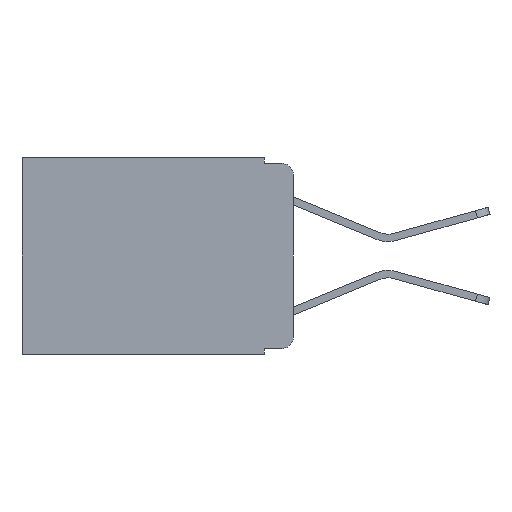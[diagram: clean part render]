
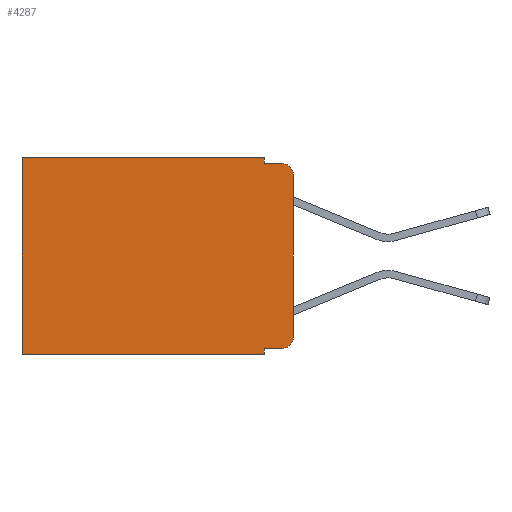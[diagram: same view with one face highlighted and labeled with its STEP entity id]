
A CAD part, left-side view. The second image highlights one B-rep face of the part: STEP entity #4287.
In plain terms, the highlighted planar face has unit normal (-1, 0, 0).
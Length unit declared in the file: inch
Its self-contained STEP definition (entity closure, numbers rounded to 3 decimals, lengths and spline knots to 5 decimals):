
#206 = CARTESIAN_POINT ( 'NONE',  ( 0.298, 0., -0.03 ) ) ;
#440 = CARTESIAN_POINT ( 'NONE',  ( 0.298, 0.051, 0. ) ) ;
#493 = VERTEX_POINT ( 'NONE', #10016 ) ;
#534 = AXIS2_PLACEMENT_3D ( 'NONE', #2322, #9544, #9946 ) ;
#638 = VECTOR ( 'NONE', #1713, 39.37008 ) ;
#674 = VECTOR ( 'NONE', #9344, 39.37008 ) ;
#797 = DIRECTION ( 'NONE',  ( 0., -1., 0. ) ) ;
#941 = DIRECTION ( 'NONE',  ( 0., 0., -1. ) ) ;
#974 = CARTESIAN_POINT ( 'NONE',  ( 0.298, 0.473, 0. ) ) ;
#1271 = EDGE_CURVE ( 'NONE', #8972, #6595, #2256, .T. ) ;
#1276 = VERTEX_POINT ( 'NONE', #10665 ) ;
#1374 = ORIENTED_EDGE ( 'NONE', *, *, #2510, .T. ) ;
#1549 = VECTOR ( 'NONE', #8406, 39.37008 ) ;
#1636 = ORIENTED_EDGE ( 'NONE', *, *, #2588, .F. ) ;
#1713 = DIRECTION ( 'NONE',  ( 0., 0., -1. ) ) ;
#1719 = VERTEX_POINT ( 'NONE', #5149 ) ;
#1764 = ORIENTED_EDGE ( 'NONE', *, *, #2994, .T. ) ;
#1784 = VERTEX_POINT ( 'NONE', #2625 ) ;
#1944 = EDGE_CURVE ( 'NONE', #493, #8972, #6693, .T. ) ;
#1969 = VECTOR ( 'NONE', #797, 39.37008 ) ;
#2031 = DIRECTION ( 'NONE',  ( 0., 0., -1. ) ) ;
#2215 = CARTESIAN_POINT ( 'NONE',  ( 0.298, 0.051, -0.01 ) ) ;
#2256 = CIRCLE ( 'NONE', #5093, 0.02 ) ;
#2265 = VERTEX_POINT ( 'NONE', #2926 ) ;
#2322 = CARTESIAN_POINT ( 'NONE',  ( 0.298, 0.02, -0.03 ) ) ;
#2338 = EDGE_CURVE ( 'NONE', #11211, #6595, #11148, .T. ) ;
#2438 = ORIENTED_EDGE ( 'NONE', *, *, #10673, .F. ) ;
#2510 = EDGE_CURVE ( 'NONE', #1276, #2265, #7933, .T. ) ;
#2533 = LINE ( 'NONE', #974, #4648 ) ;
#2588 = EDGE_CURVE ( 'NONE', #493, #5760, #6537, .T. ) ;
#2625 = CARTESIAN_POINT ( 'NONE',  ( 0.298, 0.051, -0.01 ) ) ;
#2793 = CARTESIAN_POINT ( 'NONE',  ( 0.298, 0.02, -0.333 ) ) ;
#2926 = CARTESIAN_POINT ( 'NONE',  ( 0.298, 0.473, 0. ) ) ;
#2994 = EDGE_CURVE ( 'NONE', #11211, #8817, #7641, .T. ) ;
#3105 = ORIENTED_EDGE ( 'NONE', *, *, #1271, .T. ) ;
#3228 = EDGE_CURVE ( 'NONE', #2265, #1719, #2533, .T. ) ;
#3263 = LINE ( 'NONE', #440, #638 ) ;
#3279 = CARTESIAN_POINT ( 'NONE',  ( 0.298, 0.051, 0. ) ) ;
#3442 = DIRECTION ( 'NONE',  ( 1., 0., 0. ) ) ;
#3807 = EDGE_CURVE ( 'NONE', #1276, #1784, #3263, .T. ) ;
#4073 = ORIENTED_EDGE ( 'NONE', *, *, #3807, .F. ) ;
#4240 = VECTOR ( 'NONE', #7229, 39.37008 ) ;
#4287 = ADVANCED_FACE ( 'NONE', ( #6493 ), #4765, .F. ) ;
#4389 = CARTESIAN_POINT ( 'NONE',  ( 0.298, 0., -0.343 ) ) ;
#4648 = VECTOR ( 'NONE', #941, 39.37008 ) ;
#4765 = PLANE ( 'NONE',  #7578 ) ;
#5093 = AXIS2_PLACEMENT_3D ( 'NONE', #10452, #5348, #5291 ) ;
#5149 = CARTESIAN_POINT ( 'NONE',  ( 0.298, 0.473, -0.343 ) ) ;
#5185 = EDGE_LOOP ( 'NONE', ( #7169, #1764, #8715, #4073, #1374, #8107, #2438, #1636, #5250, #3105 ) ) ;
#5250 = ORIENTED_EDGE ( 'NONE', *, *, #1944, .T. ) ;
#5254 = CARTESIAN_POINT ( 'NONE',  ( 0.298, 0., -0.313 ) ) ;
#5291 = DIRECTION ( 'NONE',  ( 0., 0., -1. ) ) ;
#5348 = DIRECTION ( 'NONE',  ( -1., 0., 0. ) ) ;
#5369 = CARTESIAN_POINT ( 'NONE',  ( 0.298, 0., 0. ) ) ;
#5760 = VERTEX_POINT ( 'NONE', #5787 ) ;
#5787 = CARTESIAN_POINT ( 'NONE',  ( 0.298, 0.051, -0.343 ) ) ;
#6493 = FACE_OUTER_BOUND ( 'NONE', #5185, .T. ) ;
#6537 = LINE ( 'NONE', #3279, #4240 ) ;
#6595 = VERTEX_POINT ( 'NONE', #5254 ) ;
#6693 = LINE ( 'NONE', #8369, #1969 ) ;
#7169 = ORIENTED_EDGE ( 'NONE', *, *, #2338, .F. ) ;
#7229 = DIRECTION ( 'NONE',  ( 0., 0., -1. ) ) ;
#7578 = AXIS2_PLACEMENT_3D ( 'NONE', #9662, #3442, #8785 ) ;
#7641 = CIRCLE ( 'NONE', #534, 0.02 ) ;
#7933 = LINE ( 'NONE', #10450, #674 ) ;
#8107 = ORIENTED_EDGE ( 'NONE', *, *, #3228, .T. ) ;
#8211 = VECTOR ( 'NONE', #9527, 39.37008 ) ;
#8369 = CARTESIAN_POINT ( 'NONE',  ( 0.298, 0.051, -0.333 ) ) ;
#8389 = LINE ( 'NONE', #2215, #1549 ) ;
#8406 = DIRECTION ( 'NONE',  ( 0., -1., 0. ) ) ;
#8715 = ORIENTED_EDGE ( 'NONE', *, *, #9162, .F. ) ;
#8785 = DIRECTION ( 'NONE',  ( 0., 0., -1. ) ) ;
#8817 = VERTEX_POINT ( 'NONE', #10238 ) ;
#8964 = VECTOR ( 'NONE', #2031, 39.37008 ) ;
#8972 = VERTEX_POINT ( 'NONE', #2793 ) ;
#9162 = EDGE_CURVE ( 'NONE', #1784, #8817, #8389, .T. ) ;
#9344 = DIRECTION ( 'NONE',  ( 0., 1., 0. ) ) ;
#9527 = DIRECTION ( 'NONE',  ( 0., 1., 0. ) ) ;
#9544 = DIRECTION ( 'NONE',  ( -1., 0., 0. ) ) ;
#9662 = CARTESIAN_POINT ( 'NONE',  ( 0.298, 0., 0. ) ) ;
#9946 = DIRECTION ( 'NONE',  ( 0., 0., -1. ) ) ;
#10016 = CARTESIAN_POINT ( 'NONE',  ( 0.298, 0.051, -0.333 ) ) ;
#10238 = CARTESIAN_POINT ( 'NONE',  ( 0.298, 0.02, -0.01 ) ) ;
#10450 = CARTESIAN_POINT ( 'NONE',  ( 0.298, 0., 0. ) ) ;
#10452 = CARTESIAN_POINT ( 'NONE',  ( 0.298, 0.02, -0.313 ) ) ;
#10665 = CARTESIAN_POINT ( 'NONE',  ( 0.298, 0.051, 0. ) ) ;
#10673 = EDGE_CURVE ( 'NONE', #5760, #1719, #10919, .T. ) ;
#10919 = LINE ( 'NONE', #4389, #8211 ) ;
#11148 = LINE ( 'NONE', #5369, #8964 ) ;
#11211 = VERTEX_POINT ( 'NONE', #206 ) ;
